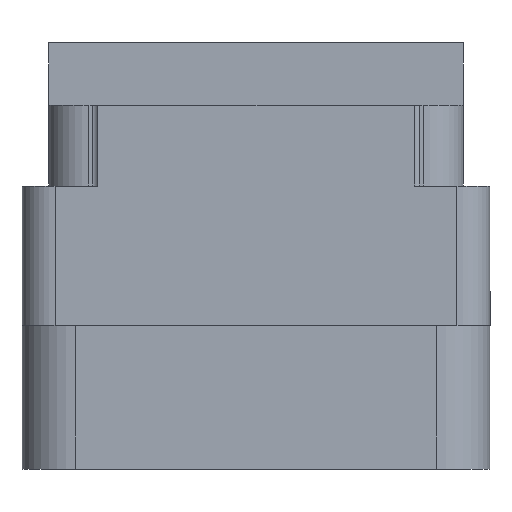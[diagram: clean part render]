
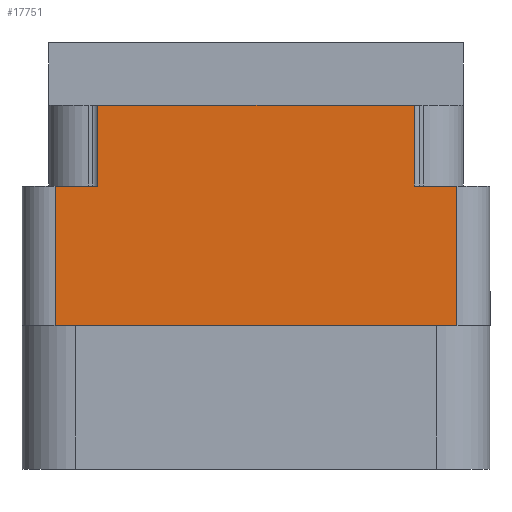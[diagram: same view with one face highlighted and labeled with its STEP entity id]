
A CAD part, left-side view. The second image highlights one B-rep face of the part: STEP entity #17751.
In plain terms, the highlighted planar face has unit normal (-1, 0, 0).
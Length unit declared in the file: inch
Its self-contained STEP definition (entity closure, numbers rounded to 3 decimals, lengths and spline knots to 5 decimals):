
#323 = DIRECTION ( 'NONE',  ( 0., -1., 0. ) ) ;
#977 = ORIENTED_EDGE ( 'NONE', *, *, #15103, .F. ) ;
#1694 = LINE ( 'NONE', #29230, #17522 ) ;
#1890 = DIRECTION ( 'NONE',  ( 0., 0., 1. ) ) ;
#2188 = CARTESIAN_POINT ( 'NONE',  ( -1., -0.376, -0.798 ) ) ;
#2724 = CARTESIAN_POINT ( 'NONE',  ( -1., 0.376, -0.529 ) ) ;
#3022 = CARTESIAN_POINT ( 'NONE',  ( -1., 0.296, -0.268 ) ) ;
#3320 = EDGE_CURVE ( 'NONE', #31687, #20657, #15476, .T. ) ;
#4825 = EDGE_CURVE ( 'NONE', #27338, #31687, #20145, .T. ) ;
#4951 = VECTOR ( 'NONE', #15385, 39.37008 ) ;
#5810 = ORIENTED_EDGE ( 'NONE', *, *, #4825, .T. ) ;
#6090 = VECTOR ( 'NONE', #28582, 39.37008 ) ;
#7391 = EDGE_CURVE ( 'NONE', #12886, #20657, #17979, .T. ) ;
#7577 = VECTOR ( 'NONE', #23573, 39.37008 ) ;
#7603 = ORIENTED_EDGE ( 'NONE', *, *, #3320, .T. ) ;
#9129 = CARTESIAN_POINT ( 'NONE',  ( -1., -0.296, -0.268 ) ) ;
#9260 = EDGE_CURVE ( 'NONE', #31235, #22179, #28311, .T. ) ;
#9759 = CARTESIAN_POINT ( 'NONE',  ( -1., -0.296, -0.117 ) ) ;
#10401 = CARTESIAN_POINT ( 'NONE',  ( -1., 0.438, -0.268 ) ) ;
#10699 = VERTEX_POINT ( 'NONE', #30603 ) ;
#11483 = FACE_OUTER_BOUND ( 'NONE', #17197, .T. ) ;
#12886 = VERTEX_POINT ( 'NONE', #9129 ) ;
#14103 = DIRECTION ( 'NONE',  ( 0., 0., 1. ) ) ;
#14494 = CARTESIAN_POINT ( 'NONE',  ( -1., 0.376, -0.798 ) ) ;
#14779 = PLANE ( 'NONE',  #15064 ) ;
#14842 = LINE ( 'NONE', #3022, #4951 ) ;
#15064 = AXIS2_PLACEMENT_3D ( 'NONE', #2188, #30145, #29926 ) ;
#15103 = EDGE_CURVE ( 'NONE', #31740, #31235, #14842, .T. ) ;
#15184 = CARTESIAN_POINT ( 'NONE',  ( -1., 0.438, -0.117 ) ) ;
#15385 = DIRECTION ( 'NONE',  ( 0., 0., 1. ) ) ;
#15476 = LINE ( 'NONE', #21028, #7577 ) ;
#16410 = EDGE_CURVE ( 'NONE', #12886, #22179, #1694, .T. ) ;
#16447 = DIRECTION ( 'NONE',  ( 0., -1., 0. ) ) ;
#16553 = CARTESIAN_POINT ( 'NONE',  ( -1., 0., -0.529 ) ) ;
#17197 = EDGE_LOOP ( 'NONE', ( #27939, #5810, #7603, #21434, #29162, #31933, #977, #28143 ) ) ;
#17522 = VECTOR ( 'NONE', #14103, 39.37008 ) ;
#17751 = ADVANCED_FACE ( 'NONE', ( #11483 ), #14779, .T. ) ;
#17979 = LINE ( 'NONE', #27949, #6090 ) ;
#20145 = LINE ( 'NONE', #16553, #29638 ) ;
#20657 = VERTEX_POINT ( 'NONE', #21124 ) ;
#21028 = CARTESIAN_POINT ( 'NONE',  ( -1., -0.376, -0.798 ) ) ;
#21124 = CARTESIAN_POINT ( 'NONE',  ( -1., -0.376, -0.268 ) ) ;
#21434 = ORIENTED_EDGE ( 'NONE', *, *, #7391, .F. ) ;
#21577 = VECTOR ( 'NONE', #25151, 39.37008 ) ;
#22179 = VERTEX_POINT ( 'NONE', #9759 ) ;
#22787 = EDGE_CURVE ( 'NONE', #27338, #10699, #23327, .T. ) ;
#23327 = LINE ( 'NONE', #14494, #25334 ) ;
#23573 = DIRECTION ( 'NONE',  ( 0., 0., 1. ) ) ;
#23951 = VECTOR ( 'NONE', #323, 39.37008 ) ;
#25151 = DIRECTION ( 'NONE',  ( 0., -1., 0. ) ) ;
#25334 = VECTOR ( 'NONE', #1890, 39.37008 ) ;
#26043 = CARTESIAN_POINT ( 'NONE',  ( -1., -0.376, -0.529 ) ) ;
#26380 = CARTESIAN_POINT ( 'NONE',  ( -1., 0.296, -0.268 ) ) ;
#27338 = VERTEX_POINT ( 'NONE', #2724 ) ;
#27939 = ORIENTED_EDGE ( 'NONE', *, *, #22787, .F. ) ;
#27949 = CARTESIAN_POINT ( 'NONE',  ( -1., -0.296, -0.268 ) ) ;
#28143 = ORIENTED_EDGE ( 'NONE', *, *, #29186, .F. ) ;
#28311 = LINE ( 'NONE', #15184, #21577 ) ;
#28582 = DIRECTION ( 'NONE',  ( 0., -1., 0. ) ) ;
#29162 = ORIENTED_EDGE ( 'NONE', *, *, #16410, .T. ) ;
#29186 = EDGE_CURVE ( 'NONE', #10699, #31740, #30275, .T. ) ;
#29230 = CARTESIAN_POINT ( 'NONE',  ( -1., -0.296, -0.268 ) ) ;
#29404 = CARTESIAN_POINT ( 'NONE',  ( -1., 0.296, -0.117 ) ) ;
#29638 = VECTOR ( 'NONE', #16447, 39.37008 ) ;
#29926 = DIRECTION ( 'NONE',  ( 0., 0., 1. ) ) ;
#30145 = DIRECTION ( 'NONE',  ( -1., 0., 0. ) ) ;
#30275 = LINE ( 'NONE', #10401, #23951 ) ;
#30603 = CARTESIAN_POINT ( 'NONE',  ( -1., 0.376, -0.268 ) ) ;
#31235 = VERTEX_POINT ( 'NONE', #29404 ) ;
#31687 = VERTEX_POINT ( 'NONE', #26043 ) ;
#31740 = VERTEX_POINT ( 'NONE', #26380 ) ;
#31933 = ORIENTED_EDGE ( 'NONE', *, *, #9260, .F. ) ;
